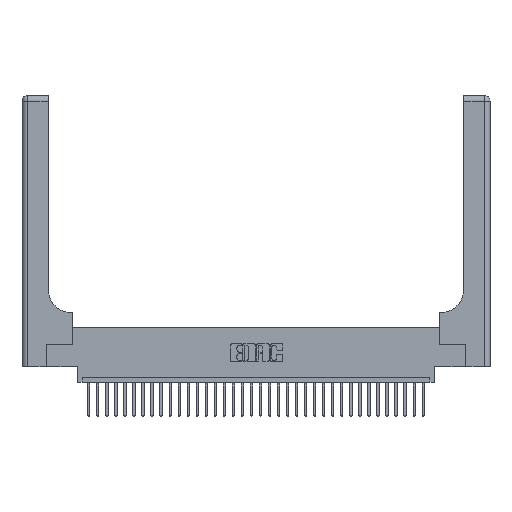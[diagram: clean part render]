
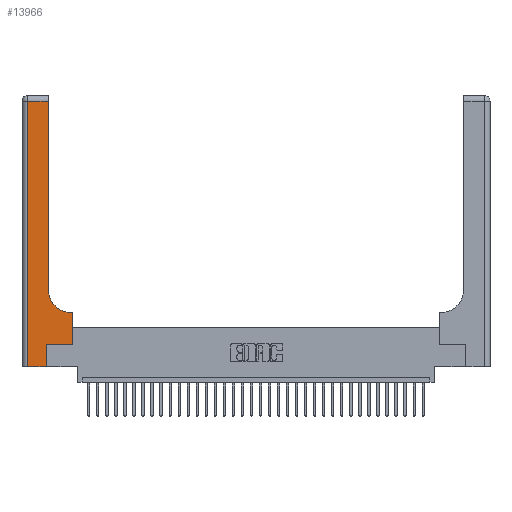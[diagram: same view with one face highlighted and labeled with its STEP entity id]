
A CAD part, top view. The second image highlights one B-rep face of the part: STEP entity #13966.
In plain terms, the highlighted planar face has unit normal (0, 0, 1).
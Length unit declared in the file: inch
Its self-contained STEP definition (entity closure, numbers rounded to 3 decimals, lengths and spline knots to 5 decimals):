
#377 = DIRECTION ( 'NONE',  ( 1., 0., 0. ) ) ;
#1094 = CARTESIAN_POINT ( 'NONE',  ( 0.2915, 0.6, 0.37 ) ) ;
#1211 = CARTESIAN_POINT ( 'NONE',  ( 0.5585, 0.25, 0.37 ) ) ;
#1306 = PLANE ( 'NONE',  #25067 ) ;
#1928 = DIRECTION ( 'NONE',  ( 1., 0., 0. ) ) ;
#2036 = CARTESIAN_POINT ( 'NONE',  ( 0.2915, 2.94, 0.37 ) ) ;
#2320 = CARTESIAN_POINT ( 'NONE',  ( 0.06, 0., 0.37 ) ) ;
#2943 = LINE ( 'NONE', #20712, #5486 ) ;
#3082 = ORIENTED_EDGE ( 'NONE', *, *, #5073, .T. ) ;
#3725 = ORIENTED_EDGE ( 'NONE', *, *, #10747, .T. ) ;
#3866 = CARTESIAN_POINT ( 'NONE',  ( 0.5585, 0.6, 0.37 ) ) ;
#3996 = VERTEX_POINT ( 'NONE', #2036 ) ;
#5073 = EDGE_CURVE ( 'NONE', #18365, #29119, #34304, .T. ) ;
#5486 = VECTOR ( 'NONE', #15478, 39.37008 ) ;
#5765 = ORIENTED_EDGE ( 'NONE', *, *, #31796, .T. ) ;
#6077 = LINE ( 'NONE', #25197, #16159 ) ;
#6486 = VERTEX_POINT ( 'NONE', #1211 ) ;
#7007 = CARTESIAN_POINT ( 'NONE',  ( 0., 2.94, 0.37 ) ) ;
#7538 = CARTESIAN_POINT ( 'NONE',  ( 0.269, 0., 0.37 ) ) ;
#7858 = CARTESIAN_POINT ( 'NONE',  ( 0.5415, 0.6, 0.37 ) ) ;
#8470 = DIRECTION ( 'NONE',  ( 0., 0., -1. ) ) ;
#8921 = ORIENTED_EDGE ( 'NONE', *, *, #18074, .T. ) ;
#8946 = DIRECTION ( 'NONE',  ( 0., 1., 0. ) ) ;
#9520 = CARTESIAN_POINT ( 'NONE',  ( 0., 3., 0.37 ) ) ;
#9910 = VECTOR ( 'NONE', #33359, 39.37008 ) ;
#10747 = EDGE_CURVE ( 'NONE', #21188, #3996, #26113, .T. ) ;
#10810 = LINE ( 'NONE', #24571, #33239 ) ;
#11065 = CARTESIAN_POINT ( 'NONE',  ( 0.2915, 0.85, 0.37 ) ) ;
#11878 = VECTOR ( 'NONE', #11992, 39.37008 ) ;
#11992 = DIRECTION ( 'NONE',  ( -1., 0., 0. ) ) ;
#12358 = CARTESIAN_POINT ( 'NONE',  ( 0.2915, 3., 0.37 ) ) ;
#12560 = ORIENTED_EDGE ( 'NONE', *, *, #13182, .T. ) ;
#13182 = EDGE_CURVE ( 'NONE', #27678, #26884, #15439, .T. ) ;
#13269 = CARTESIAN_POINT ( 'NONE',  ( 0.269, 0.25, 0.37 ) ) ;
#13858 = LINE ( 'NONE', #7007, #24269 ) ;
#13966 = ADVANCED_FACE ( 'NONE', ( #23304 ), #1306, .F. ) ;
#14396 = VECTOR ( 'NONE', #377, 39.37008 ) ;
#14644 = DIRECTION ( 'NONE',  ( -1., 0., 0. ) ) ;
#15439 = LINE ( 'NONE', #21451, #16693 ) ;
#15478 = DIRECTION ( 'NONE',  ( 0., -1., 0. ) ) ;
#15508 = DIRECTION ( 'NONE',  ( 1., 0., 0. ) ) ;
#16159 = VECTOR ( 'NONE', #33280, 39.37008 ) ;
#16693 = VECTOR ( 'NONE', #1928, 39.37008 ) ;
#18014 = EDGE_CURVE ( 'NONE', #29119, #21188, #24703, .T. ) ;
#18074 = EDGE_CURVE ( 'NONE', #29891, #27678, #2943, .T. ) ;
#18365 = VERTEX_POINT ( 'NONE', #3866 ) ;
#19407 = CARTESIAN_POINT ( 'NONE',  ( 0.269, 0.25, 0.37 ) ) ;
#20004 = DIRECTION ( 'NONE',  ( 0., 0., -1. ) ) ;
#20079 = EDGE_CURVE ( 'NONE', #3996, #29891, #13858, .T. ) ;
#20712 = CARTESIAN_POINT ( 'NONE',  ( 0.06, 3., 0.37 ) ) ;
#21188 = VERTEX_POINT ( 'NONE', #11065 ) ;
#21304 = ORIENTED_EDGE ( 'NONE', *, *, #33130, .T. ) ;
#21451 = CARTESIAN_POINT ( 'NONE',  ( 0., 0., 0.37 ) ) ;
#21513 = VERTEX_POINT ( 'NONE', #13269 ) ;
#22651 = DIRECTION ( 'NONE',  ( -1., 0., 0. ) ) ;
#23304 = FACE_OUTER_BOUND ( 'NONE', #29842, .T. ) ;
#24269 = VECTOR ( 'NONE', #14644, 39.37008 ) ;
#24571 = CARTESIAN_POINT ( 'NONE',  ( 0.5585, 0.25, 0.37 ) ) ;
#24703 = CIRCLE ( 'NONE', #28733, 0.25 ) ;
#25058 = ORIENTED_EDGE ( 'NONE', *, *, #18014, .T. ) ;
#25067 = AXIS2_PLACEMENT_3D ( 'NONE', #9520, #20004, #22651 ) ;
#25197 = CARTESIAN_POINT ( 'NONE',  ( 0.269, 0., 0.37 ) ) ;
#26113 = LINE ( 'NONE', #12358, #9910 ) ;
#26884 = VERTEX_POINT ( 'NONE', #7538 ) ;
#27678 = VERTEX_POINT ( 'NONE', #2320 ) ;
#28523 = LINE ( 'NONE', #19407, #14396 ) ;
#28733 = AXIS2_PLACEMENT_3D ( 'NONE', #29802, #8470, #15508 ) ;
#29119 = VERTEX_POINT ( 'NONE', #7858 ) ;
#29802 = CARTESIAN_POINT ( 'NONE',  ( 0.5415, 0.85, 0.37 ) ) ;
#29842 = EDGE_LOOP ( 'NONE', ( #3725, #33213, #8921, #12560, #5765, #21304, #33616, #3082, #25058 ) ) ;
#29891 = VERTEX_POINT ( 'NONE', #32538 ) ;
#29903 = EDGE_CURVE ( 'NONE', #6486, #18365, #10810, .T. ) ;
#31796 = EDGE_CURVE ( 'NONE', #26884, #21513, #6077, .T. ) ;
#32538 = CARTESIAN_POINT ( 'NONE',  ( 0.06, 2.94, 0.37 ) ) ;
#33130 = EDGE_CURVE ( 'NONE', #21513, #6486, #28523, .T. ) ;
#33213 = ORIENTED_EDGE ( 'NONE', *, *, #20079, .T. ) ;
#33239 = VECTOR ( 'NONE', #8946, 39.37008 ) ;
#33280 = DIRECTION ( 'NONE',  ( 0., 1., 0. ) ) ;
#33359 = DIRECTION ( 'NONE',  ( 0., 1., 0. ) ) ;
#33616 = ORIENTED_EDGE ( 'NONE', *, *, #29903, .T. ) ;
#34304 = LINE ( 'NONE', #1094, #11878 ) ;
